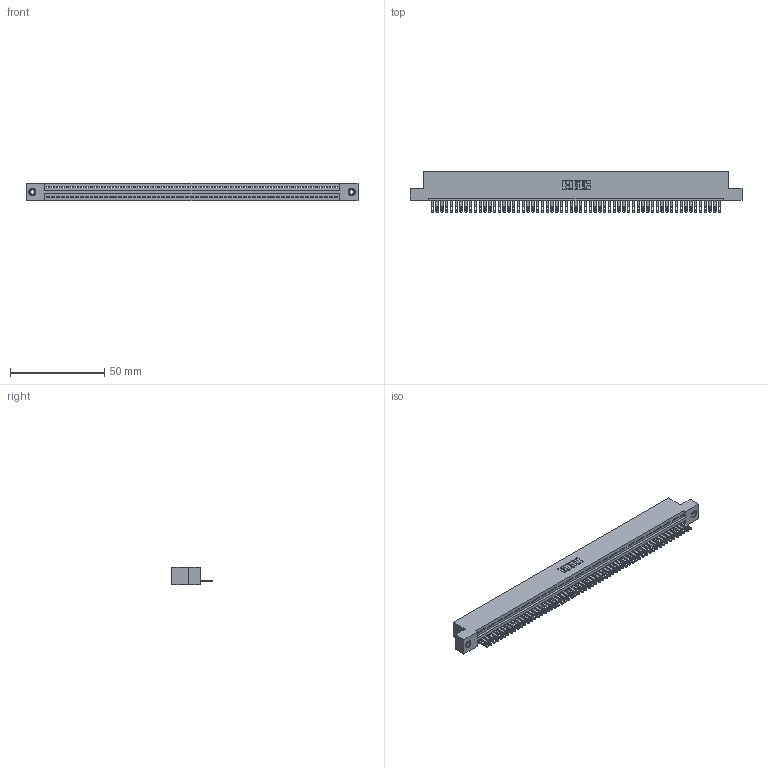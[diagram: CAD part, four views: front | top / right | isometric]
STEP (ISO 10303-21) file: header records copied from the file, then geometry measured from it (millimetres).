
FILE_DESCRIPTION (( 'STEP AP203' ), '1' );
FILE_NAME ('895-061-500-108.STEP', '2020-09-28T06:04:44', ( '' ), ( '' ), 'SwSTEP 2.0', 'SolidWorks 2020', '' );
FILE_SCHEMA (( 'CONFIG_CONTROL_DESIGN' ));
Length unit declared in the file: inch
Products named in the file (4): 345-250-001_345-250-003-102; 895-061-500-108; 845 Part_Flush Mounting Lugs - 0.156 Dia-TI; 345-292-001_345-293-100
Assembly tree (64 placements, depth 2):
  895-061-500-108
    845 Part_Flush Mounting Lugs - 0.156 Dia-TI
    345-292-001_345-293-100  x61
    345-250-001_345-250-003-102  x2
Bounding box: 176.15 x 21.51 x 9.4 mm (x, y, z)
Volume: 16917.7 mm3; surface area: 22896.4 mm2
Topology: 64 solids, 64 shells, 3480 faces, 10725 edges, 7142 vertices
Faces by surface type: plane 2186, cylinder 1278, cone 12, torus 4
Entity records: 44468 total; most frequent: CARTESIAN_POINT 7682, ORIENTED_EDGE 7670, DIRECTION 6711, EDGE_CURVE 3835, LINE 3435, VECTOR 3435, VERTEX_POINT 2552, AXIS2_PLACEMENT_3D 1638
